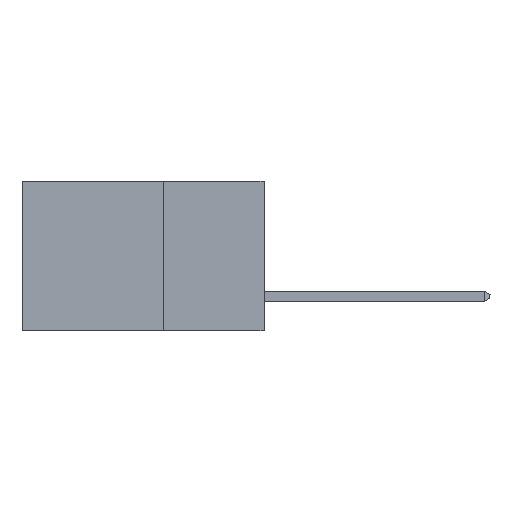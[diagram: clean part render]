
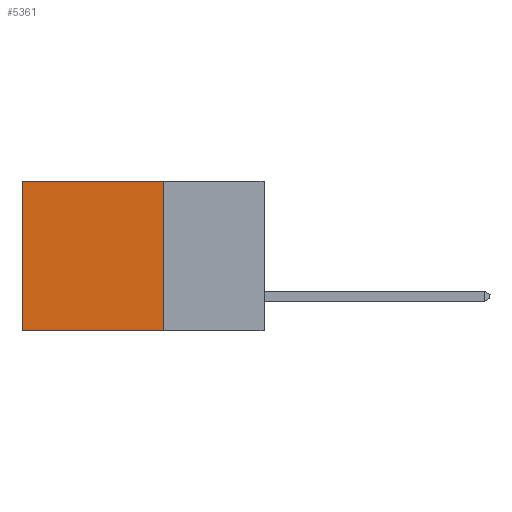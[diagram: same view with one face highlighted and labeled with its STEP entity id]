
A CAD part, left-side view. The second image highlights one B-rep face of the part: STEP entity #5361.
In plain terms, the highlighted planar face has unit normal (-1, 0, 0).
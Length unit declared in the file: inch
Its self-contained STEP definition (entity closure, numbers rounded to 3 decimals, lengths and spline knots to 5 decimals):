
#354 = CARTESIAN_POINT ( 'NONE',  ( 0.298, 0.6, -0.37 ) ) ;
#644 = VECTOR ( 'NONE', #2913, 39.37008 ) ;
#1604 = EDGE_CURVE ( 'NONE', #8147, #9436, #5509, .T. ) ;
#1847 = LINE ( 'NONE', #4786, #4495 ) ;
#2129 = ORIENTED_EDGE ( 'NONE', *, *, #8554, .T. ) ;
#2315 = CARTESIAN_POINT ( 'NONE',  ( 0.298, 0.6, 0. ) ) ;
#2913 = DIRECTION ( 'NONE',  ( 0., 0., -1. ) ) ;
#3053 = VERTEX_POINT ( 'NONE', #8674 ) ;
#3129 = EDGE_CURVE ( 'NONE', #9436, #7687, #1847, .T. ) ;
#3300 = EDGE_CURVE ( 'NONE', #3053, #7687, #5749, .T. ) ;
#3327 = FACE_OUTER_BOUND ( 'NONE', #10681, .T. ) ;
#4495 = VECTOR ( 'NONE', #11053, 39.37008 ) ;
#4786 = CARTESIAN_POINT ( 'NONE',  ( 0.298, 0.25, -0.37 ) ) ;
#4999 = VECTOR ( 'NONE', #9859, 39.37008 ) ;
#5361 = ADVANCED_FACE ( 'NONE', ( #3327 ), #6379, .F. ) ;
#5509 = LINE ( 'NONE', #8026, #644 ) ;
#5749 = LINE ( 'NONE', #2315, #10257 ) ;
#6228 = CARTESIAN_POINT ( 'NONE',  ( 0.298, 0.25, -0.37 ) ) ;
#6272 = ORIENTED_EDGE ( 'NONE', *, *, #1604, .F. ) ;
#6299 = CARTESIAN_POINT ( 'NONE',  ( 0.298, 0.25, 0. ) ) ;
#6379 = PLANE ( 'NONE',  #9375 ) ;
#7687 = VERTEX_POINT ( 'NONE', #354 ) ;
#8026 = CARTESIAN_POINT ( 'NONE',  ( 0.298, 0.25, 0. ) ) ;
#8116 = CARTESIAN_POINT ( 'NONE',  ( 0.298, 0.25, 0. ) ) ;
#8147 = VERTEX_POINT ( 'NONE', #10433 ) ;
#8554 = EDGE_CURVE ( 'NONE', #8147, #3053, #9522, .T. ) ;
#8674 = CARTESIAN_POINT ( 'NONE',  ( 0.298, 0.6, 0. ) ) ;
#8919 = DIRECTION ( 'NONE',  ( 0., 0., -1. ) ) ;
#8994 = DIRECTION ( 'NONE',  ( 1., 0., 0. ) ) ;
#9375 = AXIS2_PLACEMENT_3D ( 'NONE', #6299, #8994, #8919 ) ;
#9436 = VERTEX_POINT ( 'NONE', #6228 ) ;
#9522 = LINE ( 'NONE', #8116, #4999 ) ;
#9859 = DIRECTION ( 'NONE',  ( 0., 1., 0. ) ) ;
#10247 = DIRECTION ( 'NONE',  ( 0., 0., -1. ) ) ;
#10257 = VECTOR ( 'NONE', #10247, 39.37008 ) ;
#10337 = ORIENTED_EDGE ( 'NONE', *, *, #3129, .F. ) ;
#10433 = CARTESIAN_POINT ( 'NONE',  ( 0.298, 0.25, 0. ) ) ;
#10681 = EDGE_LOOP ( 'NONE', ( #11532, #10337, #6272, #2129 ) ) ;
#11053 = DIRECTION ( 'NONE',  ( 0., 1., 0. ) ) ;
#11532 = ORIENTED_EDGE ( 'NONE', *, *, #3300, .T. ) ;
